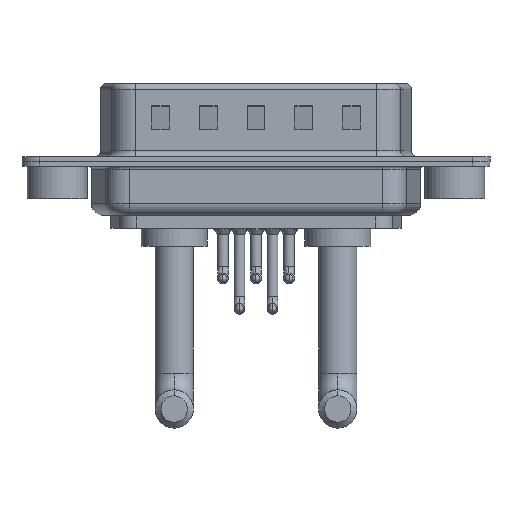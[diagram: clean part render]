
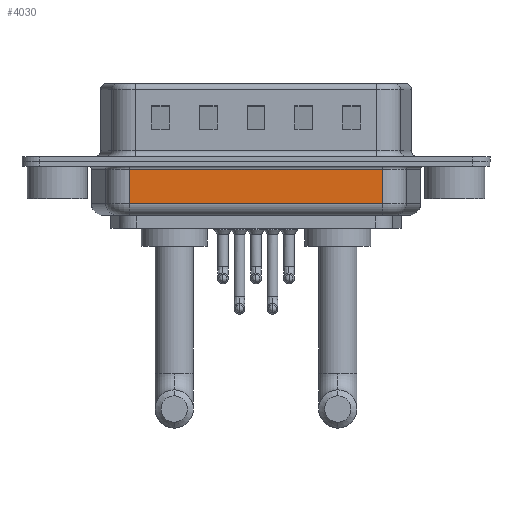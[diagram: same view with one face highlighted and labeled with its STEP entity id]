
A CAD part, front view. The second image highlights one B-rep face of the part: STEP entity #4030.
In plain terms, the highlighted planar face has unit normal (0, -1, 0).
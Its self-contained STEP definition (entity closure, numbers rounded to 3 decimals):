
#82 = EDGE_CURVE ( 'NONE', #15899, #18870, #11321, .T. ) ;
#897 = DIRECTION ( 'NONE',  ( 0., 0., 1. ) ) ;
#2114 = EDGE_LOOP ( 'NONE', ( #15024, #20353, #17323, #10534 ) ) ;
#2318 = CARTESIAN_POINT ( 'NONE',  ( 6.031, -5.35, -4.5 ) ) ;
#2563 = CARTESIAN_POINT ( 'NONE',  ( 6.031, -5.35, -4.5 ) ) ;
#2867 = DIRECTION ( 'NONE',  ( 0., 0., 1. ) ) ;
#3023 = CARTESIAN_POINT ( 'NONE',  ( 27.269, -5.35, -0.65 ) ) ;
#3581 = CARTESIAN_POINT ( 'NONE',  ( 6.031, -5.35, -3.5 ) ) ;
#3598 = AXIS2_PLACEMENT_3D ( 'NONE', #2563, #18902, #2867 ) ;
#3886 = VECTOR ( 'NONE', #6766, 1000. ) ;
#4030 = ADVANCED_FACE ( 'NONE', ( #7340 ), #7654, .F. ) ;
#5430 = CARTESIAN_POINT ( 'NONE',  ( 27.269, -5.35, -4.5 ) ) ;
#5535 = CARTESIAN_POINT ( 'NONE',  ( 6.031, -5.35, -0.65 ) ) ;
#6766 = DIRECTION ( 'NONE',  ( 1., 0., 0. ) ) ;
#7340 = FACE_OUTER_BOUND ( 'NONE', #2114, .T. ) ;
#7654 = PLANE ( 'NONE',  #3598 ) ;
#8594 = CARTESIAN_POINT ( 'NONE',  ( 27.269, -5.35, -3.5 ) ) ;
#8949 = DIRECTION ( 'NONE',  ( -1., 0., 0. ) ) ;
#10002 = LINE ( 'NONE', #2318, #11573 ) ;
#10081 = VERTEX_POINT ( 'NONE', #3023 ) ;
#10534 = ORIENTED_EDGE ( 'NONE', *, *, #12104, .T. ) ;
#11108 = CARTESIAN_POINT ( 'NONE',  ( 6.031, -5.35, -0.65 ) ) ;
#11228 = VECTOR ( 'NONE', #897, 1000. ) ;
#11321 = LINE ( 'NONE', #3581, #3886 ) ;
#11523 = VERTEX_POINT ( 'NONE', #11108 ) ;
#11573 = VECTOR ( 'NONE', #18082, 1000. ) ;
#12104 = EDGE_CURVE ( 'NONE', #10081, #11523, #12202, .T. ) ;
#12121 = CARTESIAN_POINT ( 'NONE',  ( 6.031, -5.35, -3.5 ) ) ;
#12202 = LINE ( 'NONE', #5535, #16379 ) ;
#15024 = ORIENTED_EDGE ( 'NONE', *, *, #20033, .F. ) ;
#15899 = VERTEX_POINT ( 'NONE', #12121 ) ;
#16379 = VECTOR ( 'NONE', #8949, 1000. ) ;
#16822 = LINE ( 'NONE', #5430, #11228 ) ;
#17323 = ORIENTED_EDGE ( 'NONE', *, *, #17593, .T. ) ;
#17593 = EDGE_CURVE ( 'NONE', #18870, #10081, #16822, .T. ) ;
#18082 = DIRECTION ( 'NONE',  ( 0., 0., 1. ) ) ;
#18870 = VERTEX_POINT ( 'NONE', #8594 ) ;
#18902 = DIRECTION ( 'NONE',  ( 0., 1., 0. ) ) ;
#20033 = EDGE_CURVE ( 'NONE', #15899, #11523, #10002, .T. ) ;
#20353 = ORIENTED_EDGE ( 'NONE', *, *, #82, .T. ) ;
